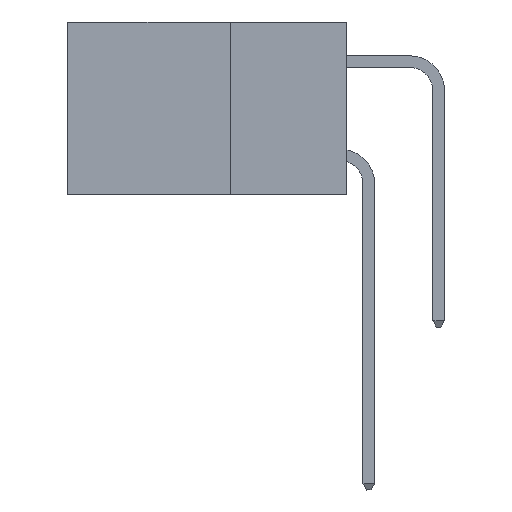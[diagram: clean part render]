
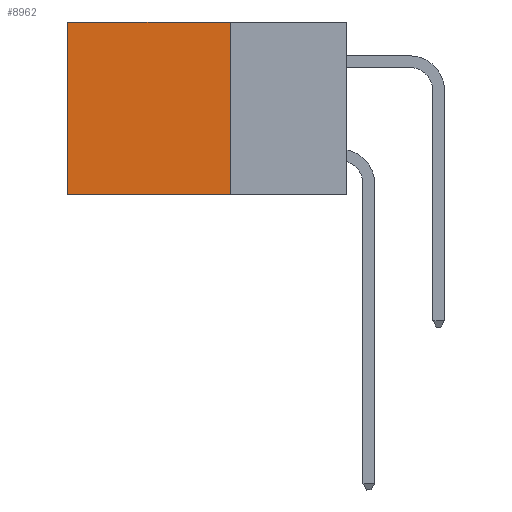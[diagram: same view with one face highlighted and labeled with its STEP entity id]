
A CAD part, left-side view. The second image highlights one B-rep face of the part: STEP entity #8962.
In plain terms, the highlighted planar face has unit normal (-1, 0, 0).
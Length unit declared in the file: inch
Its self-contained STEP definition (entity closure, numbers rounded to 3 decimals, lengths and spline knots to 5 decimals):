
#821 = CARTESIAN_POINT ( 'NONE',  ( 0.2875, 0.25, 0. ) ) ;
#838 = ORIENTED_EDGE ( 'NONE', *, *, #28558, .T. ) ;
#845 = VERTEX_POINT ( 'NONE', #22124 ) ;
#1291 = DIRECTION ( 'NONE',  ( 0., 1., 0. ) ) ;
#2471 = ORIENTED_EDGE ( 'NONE', *, *, #29070, .T. ) ;
#2986 = DIRECTION ( 'NONE',  ( 0., 0., -1. ) ) ;
#3274 = VERTEX_POINT ( 'NONE', #821 ) ;
#3455 = PLANE ( 'NONE',  #14354 ) ;
#5604 = ORIENTED_EDGE ( 'NONE', *, *, #27455, .F. ) ;
#5612 = VECTOR ( 'NONE', #25299, 39.37008 ) ;
#6843 = ORIENTED_EDGE ( 'NONE', *, *, #19784, .F. ) ;
#7762 = FACE_OUTER_BOUND ( 'NONE', #10774, .T. ) ;
#8962 = ADVANCED_FACE ( 'NONE', ( #7762 ), #3455, .F. ) ;
#9194 = VECTOR ( 'NONE', #1291, 39.37008 ) ;
#9560 = CARTESIAN_POINT ( 'NONE',  ( 0.2875, 0.25, -0.37 ) ) ;
#9725 = LINE ( 'NONE', #10636, #17686 ) ;
#10443 = CARTESIAN_POINT ( 'NONE',  ( 0.2875, 0.25, 0. ) ) ;
#10636 = CARTESIAN_POINT ( 'NONE',  ( 0.2875, 0.25, 0. ) ) ;
#10774 = EDGE_LOOP ( 'NONE', ( #838, #6843, #5604, #2471 ) ) ;
#12489 = CARTESIAN_POINT ( 'NONE',  ( 0.2875, 0.25, -0.37 ) ) ;
#12616 = VERTEX_POINT ( 'NONE', #26804 ) ;
#14354 = AXIS2_PLACEMENT_3D ( 'NONE', #10443, #17251, #26899 ) ;
#15192 = DIRECTION ( 'NONE',  ( 0., 0., -1. ) ) ;
#17251 = DIRECTION ( 'NONE',  ( 1., 0., 0. ) ) ;
#17686 = VECTOR ( 'NONE', #15192, 39.37008 ) ;
#17949 = LINE ( 'NONE', #25102, #5612 ) ;
#18111 = VERTEX_POINT ( 'NONE', #9560 ) ;
#19784 = EDGE_CURVE ( 'NONE', #18111, #845, #29895, .T. ) ;
#22124 = CARTESIAN_POINT ( 'NONE',  ( 0.2875, 0.6, -0.37 ) ) ;
#24163 = VECTOR ( 'NONE', #2986, 39.37008 ) ;
#25102 = CARTESIAN_POINT ( 'NONE',  ( 0.2875, 0.25, 0. ) ) ;
#25299 = DIRECTION ( 'NONE',  ( 0., 1., 0. ) ) ;
#25977 = LINE ( 'NONE', #28886, #24163 ) ;
#26804 = CARTESIAN_POINT ( 'NONE',  ( 0.2875, 0.6, 0. ) ) ;
#26899 = DIRECTION ( 'NONE',  ( 0., 0., -1. ) ) ;
#27455 = EDGE_CURVE ( 'NONE', #3274, #18111, #9725, .T. ) ;
#28558 = EDGE_CURVE ( 'NONE', #12616, #845, #25977, .T. ) ;
#28886 = CARTESIAN_POINT ( 'NONE',  ( 0.2875, 0.6, 0. ) ) ;
#29070 = EDGE_CURVE ( 'NONE', #3274, #12616, #17949, .T. ) ;
#29895 = LINE ( 'NONE', #12489, #9194 ) ;
